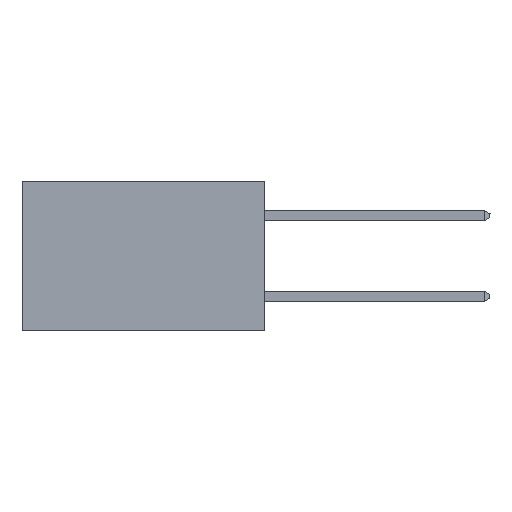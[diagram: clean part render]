
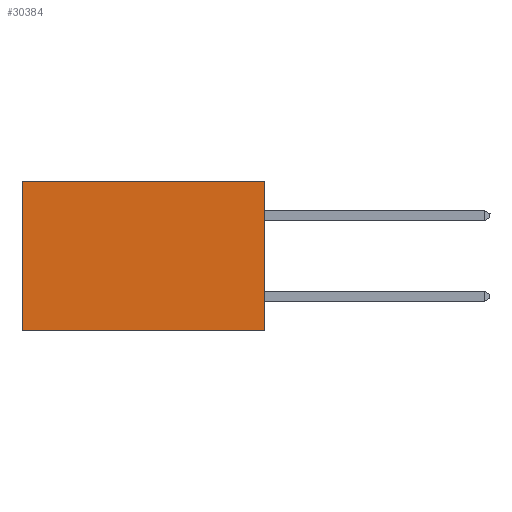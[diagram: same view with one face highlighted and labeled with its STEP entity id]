
A CAD part, left-side view. The second image highlights one B-rep face of the part: STEP entity #30384.
In plain terms, the highlighted planar face has unit normal (-1, 0, 0).
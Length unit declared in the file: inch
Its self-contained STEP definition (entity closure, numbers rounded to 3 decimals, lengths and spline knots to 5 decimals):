
#641 = VERTEX_POINT ( 'NONE', #13668 ) ;
#1386 = DIRECTION ( 'NONE',  ( 1., 0., 0. ) ) ;
#2347 = ORIENTED_EDGE ( 'NONE', *, *, #7446, .T. ) ;
#3493 = VECTOR ( 'NONE', #6036, 39.37008 ) ;
#3518 = VERTEX_POINT ( 'NONE', #20692 ) ;
#4250 = LINE ( 'NONE', #17975, #3493 ) ;
#6036 = DIRECTION ( 'NONE',  ( 0., 0., -1. ) ) ;
#6362 = EDGE_LOOP ( 'NONE', ( #30279, #13097, #10956, #2347 ) ) ;
#7399 = DIRECTION ( 'NONE',  ( 0., 0., -1. ) ) ;
#7446 = EDGE_CURVE ( 'NONE', #3518, #28956, #18535, .T. ) ;
#7509 = FACE_OUTER_BOUND ( 'NONE', #6362, .T. ) ;
#7841 = CARTESIAN_POINT ( 'NONE',  ( 0.298, 0., -0.37 ) ) ;
#9658 = AXIS2_PLACEMENT_3D ( 'NONE', #15742, #1386, #18171 ) ;
#10956 = ORIENTED_EDGE ( 'NONE', *, *, #13030, .F. ) ;
#11328 = VECTOR ( 'NONE', #7399, 39.37008 ) ;
#12137 = VECTOR ( 'NONE', #12482, 39.37008 ) ;
#12482 = DIRECTION ( 'NONE',  ( 0., 1., 0. ) ) ;
#12648 = EDGE_CURVE ( 'NONE', #28956, #16180, #4250, .T. ) ;
#13030 = EDGE_CURVE ( 'NONE', #3518, #641, #24836, .T. ) ;
#13097 = ORIENTED_EDGE ( 'NONE', *, *, #23716, .F. ) ;
#13668 = CARTESIAN_POINT ( 'NONE',  ( 0.298, 0., -0.37 ) ) ;
#15742 = CARTESIAN_POINT ( 'NONE',  ( 0.298, 0., 0. ) ) ;
#16180 = VERTEX_POINT ( 'NONE', #17576 ) ;
#17576 = CARTESIAN_POINT ( 'NONE',  ( 0.298, 0.6, -0.37 ) ) ;
#17975 = CARTESIAN_POINT ( 'NONE',  ( 0.298, 0.6, 0. ) ) ;
#18070 = PLANE ( 'NONE',  #9658 ) ;
#18171 = DIRECTION ( 'NONE',  ( 0., 0., -1. ) ) ;
#18535 = LINE ( 'NONE', #21542, #12137 ) ;
#18544 = VECTOR ( 'NONE', #24458, 39.37008 ) ;
#20692 = CARTESIAN_POINT ( 'NONE',  ( 0.298, 0., 0. ) ) ;
#21542 = CARTESIAN_POINT ( 'NONE',  ( 0.298, 0., 0. ) ) ;
#21641 = CARTESIAN_POINT ( 'NONE',  ( 0.298, 0., 0. ) ) ;
#22797 = CARTESIAN_POINT ( 'NONE',  ( 0.298, 0.6, 0. ) ) ;
#23716 = EDGE_CURVE ( 'NONE', #641, #16180, #24893, .T. ) ;
#24458 = DIRECTION ( 'NONE',  ( 0., 1., 0. ) ) ;
#24836 = LINE ( 'NONE', #21641, #11328 ) ;
#24893 = LINE ( 'NONE', #7841, #18544 ) ;
#28956 = VERTEX_POINT ( 'NONE', #22797 ) ;
#30279 = ORIENTED_EDGE ( 'NONE', *, *, #12648, .T. ) ;
#30384 = ADVANCED_FACE ( 'NONE', ( #7509 ), #18070, .F. ) ;
